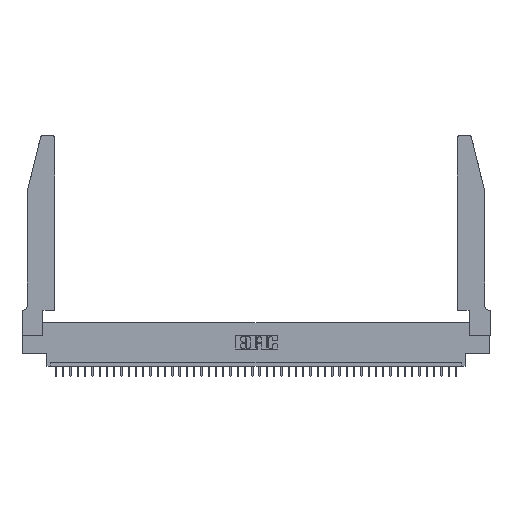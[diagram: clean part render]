
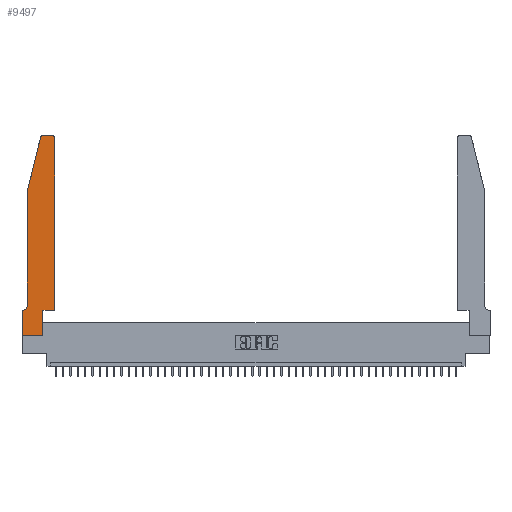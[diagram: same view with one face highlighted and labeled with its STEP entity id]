
A CAD part, top view. The second image highlights one B-rep face of the part: STEP entity #9497.
In plain terms, the highlighted planar face has unit normal (0, 0, 1).
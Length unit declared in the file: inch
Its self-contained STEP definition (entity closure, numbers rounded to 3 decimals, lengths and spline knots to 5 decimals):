
#234 = VERTEX_POINT ( 'NONE', #26771 ) ;
#584 = VERTEX_POINT ( 'NONE', #12514 ) ;
#619 = EDGE_CURVE ( 'NONE', #12830, #13900, #34093, .T. ) ;
#791 = CARTESIAN_POINT ( 'NONE',  ( 0.0055, 0.42, 0.37 ) ) ;
#1735 = CARTESIAN_POINT ( 'NONE',  ( 0.2865, 0.35, 0.37 ) ) ;
#2245 = EDGE_CURVE ( 'NONE', #22160, #13305, #15679, .T. ) ;
#2459 = CARTESIAN_POINT ( 'NONE',  ( 0.284, 2.72, 0.37 ) ) ;
#2544 = VERTEX_POINT ( 'NONE', #41523 ) ;
#2683 = EDGE_CURVE ( 'NONE', #35360, #9013, #15950, .T. ) ;
#3137 = DIRECTION ( 'NONE',  ( 1., 0., 0. ) ) ;
#3541 = VECTOR ( 'NONE', #16881, 39.37008 ) ;
#3803 = CARTESIAN_POINT ( 'NONE',  ( 0.4505, 0.35, 0.37 ) ) ;
#4853 = EDGE_CURVE ( 'NONE', #2544, #12830, #23351, .T. ) ;
#4993 = ORIENTED_EDGE ( 'NONE', *, *, #41642, .T. ) ;
#5143 = LINE ( 'NONE', #18434, #7191 ) ;
#5959 = CARTESIAN_POINT ( 'NONE',  ( 0., 0.35, 0.37 ) ) ;
#6578 = EDGE_CURVE ( 'NONE', #13305, #27429, #26736, .T. ) ;
#7191 = VECTOR ( 'NONE', #21869, 39.37008 ) ;
#7445 = DIRECTION ( 'NONE',  ( 1., 0., 0. ) ) ;
#7713 = ORIENTED_EDGE ( 'NONE', *, *, #619, .T. ) ;
#8026 = AXIS2_PLACEMENT_3D ( 'NONE', #38364, #11097, #7445 ) ;
#8617 = CARTESIAN_POINT ( 'NONE',  ( 0.2865, 0., 0.37 ) ) ;
#8930 = EDGE_CURVE ( 'NONE', #584, #22160, #12199, .T. ) ;
#9013 = VERTEX_POINT ( 'NONE', #12872 ) ;
#9497 = ADVANCED_FACE ( 'NONE', ( #23821 ), #40761, .T. ) ;
#9836 = DIRECTION ( 'NONE',  ( 0., 0., 1. ) ) ;
#10635 = CARTESIAN_POINT ( 'NONE',  ( 0.4505, 2.72, 0.37 ) ) ;
#10882 = EDGE_CURVE ( 'NONE', #27429, #11361, #23085, .T. ) ;
#11097 = DIRECTION ( 'NONE',  ( 0., 0., 1. ) ) ;
#11260 = CARTESIAN_POINT ( 'NONE',  ( 0.0755, 0.35, 0.37 ) ) ;
#11294 = DIRECTION ( 'NONE',  ( 0., 0., -1. ) ) ;
#11361 = VERTEX_POINT ( 'NONE', #10635 ) ;
#11412 = DIRECTION ( 'NONE',  ( 0., -1., 0. ) ) ;
#12022 = CARTESIAN_POINT ( 'NONE',  ( 0.0755, 0.42, 0.37 ) ) ;
#12199 = LINE ( 'NONE', #29405, #16426 ) ;
#12259 = VECTOR ( 'NONE', #40187, 39.37008 ) ;
#12514 = CARTESIAN_POINT ( 'NONE',  ( 0., 0., 0.37 ) ) ;
#12830 = VERTEX_POINT ( 'NONE', #17984 ) ;
#12872 = CARTESIAN_POINT ( 'NONE',  ( 0.0055, 0.35, 0.37 ) ) ;
#12879 = AXIS2_PLACEMENT_3D ( 'NONE', #2459, #23955, #16847 ) ;
#13305 = VERTEX_POINT ( 'NONE', #22963 ) ;
#13543 = ORIENTED_EDGE ( 'NONE', *, *, #2245, .T. ) ;
#13900 = VERTEX_POINT ( 'NONE', #41816 ) ;
#14500 = ORIENTED_EDGE ( 'NONE', *, *, #21123, .T. ) ;
#15679 = LINE ( 'NONE', #1735, #12259 ) ;
#15860 = DIRECTION ( 'NONE',  ( 1., 0., 0. ) ) ;
#15910 = VECTOR ( 'NONE', #3137, 39.37008 ) ;
#15950 = CIRCLE ( 'NONE', #35665, 0.07 ) ;
#16426 = VECTOR ( 'NONE', #15860, 39.37008 ) ;
#16847 = DIRECTION ( 'NONE',  ( 1., 0., 0. ) ) ;
#16881 = DIRECTION ( 'NONE',  ( 0., 1., 0. ) ) ;
#17657 = ORIENTED_EDGE ( 'NONE', *, *, #27363, .T. ) ;
#17984 = CARTESIAN_POINT ( 'NONE',  ( 0.284, 2.75, 0.37 ) ) ;
#18434 = CARTESIAN_POINT ( 'NONE',  ( 0.0755, 2., 0.37 ) ) ;
#19830 = EDGE_CURVE ( 'NONE', #9013, #234, #42642, .T. ) ;
#20249 = EDGE_LOOP ( 'NONE', ( #38620, #7713, #14500, #4993, #39390, #28721, #43834, #25184, #13543, #40021, #34265, #17657 ) ) ;
#20342 = CARTESIAN_POINT ( 'NONE',  ( 0.2605, 2.75, 0.37 ) ) ;
#21123 = EDGE_CURVE ( 'NONE', #13900, #27430, #31887, .T. ) ;
#21869 = DIRECTION ( 'NONE',  ( 0., -1., 0. ) ) ;
#22160 = VERTEX_POINT ( 'NONE', #8617 ) ;
#22963 = CARTESIAN_POINT ( 'NONE',  ( 0.2865, 0.35, 0.37 ) ) ;
#23085 = LINE ( 'NONE', #30200, #3541 ) ;
#23351 = LINE ( 'NONE', #20342, #38111 ) ;
#23821 = FACE_OUTER_BOUND ( 'NONE', #20249, .T. ) ;
#23955 = DIRECTION ( 'NONE',  ( 0., 0., 1. ) ) ;
#23973 = CARTESIAN_POINT ( 'NONE',  ( 0.4505, 0.35, 0.37 ) ) ;
#24324 = EDGE_CURVE ( 'NONE', #234, #584, #32719, .T. ) ;
#25184 = ORIENTED_EDGE ( 'NONE', *, *, #8930, .T. ) ;
#25248 = DIRECTION ( 'NONE',  ( -1., 0., 0. ) ) ;
#25279 = DIRECTION ( 'NONE',  ( -1., 0., 0. ) ) ;
#26736 = LINE ( 'NONE', #23973, #15910 ) ;
#26771 = CARTESIAN_POINT ( 'NONE',  ( 0., 0.35, 0.37 ) ) ;
#27363 = EDGE_CURVE ( 'NONE', #11361, #2544, #27771, .T. ) ;
#27429 = VERTEX_POINT ( 'NONE', #3803 ) ;
#27430 = VERTEX_POINT ( 'NONE', #31729 ) ;
#27771 = CIRCLE ( 'NONE', #8026, 0.03 ) ;
#28345 = VECTOR ( 'NONE', #25248, 39.37008 ) ;
#28721 = ORIENTED_EDGE ( 'NONE', *, *, #19830, .T. ) ;
#29364 = DIRECTION ( 'NONE',  ( -0.239, -0.971, 0. ) ) ;
#29405 = CARTESIAN_POINT ( 'NONE',  ( 0., 0., 0.37 ) ) ;
#30200 = CARTESIAN_POINT ( 'NONE',  ( 0.4505, 0.35, 0.37 ) ) ;
#31729 = CARTESIAN_POINT ( 'NONE',  ( 0.0755, 2., 0.37 ) ) ;
#31887 = LINE ( 'NONE', #32339, #36312 ) ;
#32339 = CARTESIAN_POINT ( 'NONE',  ( 0.0755, 2., 0.37 ) ) ;
#32719 = LINE ( 'NONE', #43692, #40925 ) ;
#33173 = AXIS2_PLACEMENT_3D ( 'NONE', #5959, #9836, #37773 ) ;
#34093 = CIRCLE ( 'NONE', #12879, 0.03 ) ;
#34265 = ORIENTED_EDGE ( 'NONE', *, *, #10882, .T. ) ;
#35360 = VERTEX_POINT ( 'NONE', #12022 ) ;
#35665 = AXIS2_PLACEMENT_3D ( 'NONE', #791, #11294, #25279 ) ;
#36312 = VECTOR ( 'NONE', #29364, 39.37008 ) ;
#37308 = DIRECTION ( 'NONE',  ( -1., 0., 0. ) ) ;
#37773 = DIRECTION ( 'NONE',  ( 1., 0., 0. ) ) ;
#38111 = VECTOR ( 'NONE', #37308, 39.37008 ) ;
#38364 = CARTESIAN_POINT ( 'NONE',  ( 0.4205, 2.72, 0.37 ) ) ;
#38620 = ORIENTED_EDGE ( 'NONE', *, *, #4853, .T. ) ;
#39390 = ORIENTED_EDGE ( 'NONE', *, *, #2683, .T. ) ;
#40021 = ORIENTED_EDGE ( 'NONE', *, *, #6578, .T. ) ;
#40187 = DIRECTION ( 'NONE',  ( 0., 1., 0. ) ) ;
#40761 = PLANE ( 'NONE',  #33173 ) ;
#40925 = VECTOR ( 'NONE', #11412, 39.37008 ) ;
#41523 = CARTESIAN_POINT ( 'NONE',  ( 0.4205, 2.75, 0.37 ) ) ;
#41642 = EDGE_CURVE ( 'NONE', #27430, #35360, #5143, .T. ) ;
#41816 = CARTESIAN_POINT ( 'NONE',  ( 0.25487, 2.72718, 0.37 ) ) ;
#42642 = LINE ( 'NONE', #11260, #28345 ) ;
#43692 = CARTESIAN_POINT ( 'NONE',  ( 0., 0., 0.37 ) ) ;
#43834 = ORIENTED_EDGE ( 'NONE', *, *, #24324, .T. ) ;
